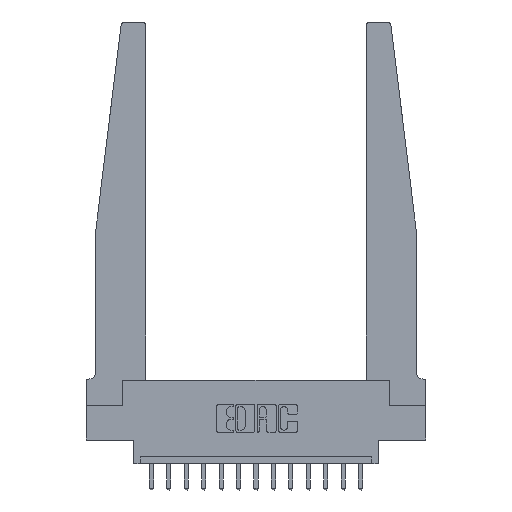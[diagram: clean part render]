
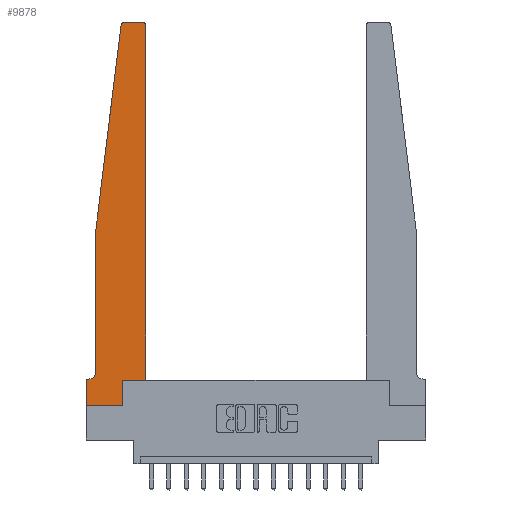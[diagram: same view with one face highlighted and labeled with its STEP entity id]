
A CAD part, top view. The second image highlights one B-rep face of the part: STEP entity #9878.
In plain terms, the highlighted planar face has unit normal (0, 0, 1).
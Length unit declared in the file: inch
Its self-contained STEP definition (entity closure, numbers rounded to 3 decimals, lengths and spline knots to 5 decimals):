
#317 = LINE ( 'NONE', #16357, #6888 ) ;
#931 = CARTESIAN_POINT ( 'NONE',  ( 0.015, 0.1875, 0.37 ) ) ;
#975 = EDGE_CURVE ( 'NONE', #17416, #9351, #16447, .T. ) ;
#1007 = DIRECTION ( 'NONE',  ( 1., 0., 0. ) ) ;
#1356 = VERTEX_POINT ( 'NONE', #2754 ) ;
#1375 = EDGE_CURVE ( 'NONE', #9351, #11897, #11931, .T. ) ;
#1663 = DIRECTION ( 'NONE',  ( -1., 0., 0. ) ) ;
#1745 = DIRECTION ( 'NONE',  ( 0., 0., -1. ) ) ;
#1753 = DIRECTION ( 'NONE',  ( 0., 0., 1. ) ) ;
#1827 = ORIENTED_EDGE ( 'NONE', *, *, #7842, .T. ) ;
#1927 = EDGE_CURVE ( 'NONE', #10220, #7853, #13602, .T. ) ;
#1990 = DIRECTION ( 'NONE',  ( 1., 0., 0. ) ) ;
#2330 = DIRECTION ( 'NONE',  ( 0., -1., 0. ) ) ;
#2385 = VERTEX_POINT ( 'NONE', #12582 ) ;
#2676 = EDGE_LOOP ( 'NONE', ( #6490, #8940, #11402, #15513, #10098, #4180, #11058, #1827, #3292, #8039, #5232, #17173 ) ) ;
#2754 = CARTESIAN_POINT ( 'NONE',  ( 0.425, 0.18, 0.37 ) ) ;
#2849 = VERTEX_POINT ( 'NONE', #7495 ) ;
#2889 = CARTESIAN_POINT ( 'NONE',  ( 0.2605, 0.18, 0.37 ) ) ;
#3292 = ORIENTED_EDGE ( 'NONE', *, *, #6015, .T. ) ;
#4180 = ORIENTED_EDGE ( 'NONE', *, *, #13503, .T. ) ;
#4207 = DIRECTION ( 'NONE',  ( 0., 1., 0. ) ) ;
#4223 = LINE ( 'NONE', #2889, #10040 ) ;
#4367 = VECTOR ( 'NONE', #1007, 39.37008 ) ;
#4486 = VERTEX_POINT ( 'NONE', #10503 ) ;
#4668 = FACE_OUTER_BOUND ( 'NONE', #2676, .T. ) ;
#5232 = ORIENTED_EDGE ( 'NONE', *, *, #15685, .T. ) ;
#5242 = DIRECTION ( 'NONE',  ( -1., 0., 0. ) ) ;
#5994 = AXIS2_PLACEMENT_3D ( 'NONE', #13742, #1745, #1663 ) ;
#6015 = EDGE_CURVE ( 'NONE', #2849, #12527, #4223, .T. ) ;
#6255 = CARTESIAN_POINT ( 'NONE',  ( 0.065, 1.25, 0.37 ) ) ;
#6296 = DIRECTION ( 'NONE',  ( 0., 0., 1. ) ) ;
#6426 = LINE ( 'NONE', #10212, #15548 ) ;
#6455 = DIRECTION ( 'NONE',  ( -0.122, -0.992, 0. ) ) ;
#6490 = ORIENTED_EDGE ( 'NONE', *, *, #13699, .T. ) ;
#6590 = EDGE_CURVE ( 'NONE', #4486, #8079, #13773, .T. ) ;
#6725 = CARTESIAN_POINT ( 'NONE',  ( 0.25, 2.75, 0.37 ) ) ;
#6888 = VECTOR ( 'NONE', #4207, 39.37008 ) ;
#7177 = CARTESIAN_POINT ( 'NONE',  ( 0., 0., 0.37 ) ) ;
#7495 = CARTESIAN_POINT ( 'NONE',  ( 0.2605, 0., 0.37 ) ) ;
#7842 = EDGE_CURVE ( 'NONE', #2385, #2849, #11161, .T. ) ;
#7853 = VERTEX_POINT ( 'NONE', #931 ) ;
#7958 = EDGE_CURVE ( 'NONE', #17322, #2385, #11512, .T. ) ;
#8039 = ORIENTED_EDGE ( 'NONE', *, *, #15219, .T. ) ;
#8075 = DIRECTION ( 'NONE',  ( -1., 0., 0. ) ) ;
#8079 = VERTEX_POINT ( 'NONE', #10423 ) ;
#8200 = AXIS2_PLACEMENT_3D ( 'NONE', #8365, #1753, #14012 ) ;
#8219 = DIRECTION ( 'NONE',  ( 1., 0., 0. ) ) ;
#8365 = CARTESIAN_POINT ( 'NONE',  ( 0., 0.1875, 0.37 ) ) ;
#8443 = VECTOR ( 'NONE', #1990, 39.37008 ) ;
#8846 = CARTESIAN_POINT ( 'NONE',  ( 0.425, 0.18, 0.37 ) ) ;
#8940 = ORIENTED_EDGE ( 'NONE', *, *, #975, .T. ) ;
#9100 = VECTOR ( 'NONE', #8075, 39.37008 ) ;
#9351 = VERTEX_POINT ( 'NONE', #9607 ) ;
#9607 = CARTESIAN_POINT ( 'NONE',  ( 0.24675, 2.72367, 0.37 ) ) ;
#9849 = PLANE ( 'NONE',  #8200 ) ;
#9878 = ADVANCED_FACE ( 'NONE', ( #4668 ), #9849, .T. ) ;
#9993 = EDGE_CURVE ( 'NONE', #11897, #10220, #6426, .T. ) ;
#10040 = VECTOR ( 'NONE', #16294, 39.37008 ) ;
#10098 = ORIENTED_EDGE ( 'NONE', *, *, #1927, .T. ) ;
#10212 = CARTESIAN_POINT ( 'NONE',  ( 0.065, 1.25, 0.37 ) ) ;
#10220 = VERTEX_POINT ( 'NONE', #10886 ) ;
#10389 = DIRECTION ( 'NONE',  ( 0., -1., 0. ) ) ;
#10423 = CARTESIAN_POINT ( 'NONE',  ( 0.395, 2.75, 0.37 ) ) ;
#10503 = CARTESIAN_POINT ( 'NONE',  ( 0.425, 2.72, 0.37 ) ) ;
#10886 = CARTESIAN_POINT ( 'NONE',  ( 0.065, 0.2375, 0.37 ) ) ;
#10997 = VECTOR ( 'NONE', #2330, 39.37008 ) ;
#11058 = ORIENTED_EDGE ( 'NONE', *, *, #7958, .T. ) ;
#11161 = LINE ( 'NONE', #7177, #8443 ) ;
#11402 = ORIENTED_EDGE ( 'NONE', *, *, #1375, .T. ) ;
#11512 = LINE ( 'NONE', #16885, #10997 ) ;
#11515 = CARTESIAN_POINT ( 'NONE',  ( 0.2605, 0.18, 0.37 ) ) ;
#11897 = VERTEX_POINT ( 'NONE', #6255 ) ;
#11931 = LINE ( 'NONE', #16062, #14258 ) ;
#12038 = CARTESIAN_POINT ( 'NONE',  ( 0., 0.1875, 0.37 ) ) ;
#12291 = DIRECTION ( 'NONE',  ( 0., 0., 1. ) ) ;
#12317 = LINE ( 'NONE', #16362, #9100 ) ;
#12465 = CARTESIAN_POINT ( 'NONE',  ( 0.27653, 2.75, 0.37 ) ) ;
#12527 = VERTEX_POINT ( 'NONE', #11515 ) ;
#12582 = CARTESIAN_POINT ( 'NONE',  ( 0., 0., 0.37 ) ) ;
#13362 = CARTESIAN_POINT ( 'NONE',  ( 0.27653, 2.72, 0.37 ) ) ;
#13503 = EDGE_CURVE ( 'NONE', #7853, #17322, #12317, .T. ) ;
#13602 = CIRCLE ( 'NONE', #5994, 0.05 ) ;
#13610 = LINE ( 'NONE', #6725, #15887 ) ;
#13699 = EDGE_CURVE ( 'NONE', #8079, #17416, #13610, .T. ) ;
#13742 = CARTESIAN_POINT ( 'NONE',  ( 0.015, 0.2375, 0.37 ) ) ;
#13773 = CIRCLE ( 'NONE', #14621, 0.03 ) ;
#13794 = CARTESIAN_POINT ( 'NONE',  ( 0.395, 2.72, 0.37 ) ) ;
#14012 = DIRECTION ( 'NONE',  ( 1., 0., 0. ) ) ;
#14236 = DIRECTION ( 'NONE',  ( 1., 0., 0. ) ) ;
#14258 = VECTOR ( 'NONE', #6455, 39.37008 ) ;
#14621 = AXIS2_PLACEMENT_3D ( 'NONE', #13794, #6296, #14236 ) ;
#15219 = EDGE_CURVE ( 'NONE', #12527, #1356, #16962, .T. ) ;
#15337 = AXIS2_PLACEMENT_3D ( 'NONE', #13362, #12291, #8219 ) ;
#15513 = ORIENTED_EDGE ( 'NONE', *, *, #9993, .T. ) ;
#15548 = VECTOR ( 'NONE', #10389, 39.37008 ) ;
#15685 = EDGE_CURVE ( 'NONE', #1356, #4486, #317, .T. ) ;
#15887 = VECTOR ( 'NONE', #5242, 39.37008 ) ;
#16062 = CARTESIAN_POINT ( 'NONE',  ( 0.065, 1.25, 0.37 ) ) ;
#16294 = DIRECTION ( 'NONE',  ( 0., 1., 0. ) ) ;
#16357 = CARTESIAN_POINT ( 'NONE',  ( 0.425, 0.18, 0.37 ) ) ;
#16362 = CARTESIAN_POINT ( 'NONE',  ( 0.065, 0.1875, 0.37 ) ) ;
#16447 = CIRCLE ( 'NONE', #15337, 0.03 ) ;
#16885 = CARTESIAN_POINT ( 'NONE',  ( 0., 0., 0.37 ) ) ;
#16962 = LINE ( 'NONE', #8846, #4367 ) ;
#17173 = ORIENTED_EDGE ( 'NONE', *, *, #6590, .T. ) ;
#17322 = VERTEX_POINT ( 'NONE', #12038 ) ;
#17416 = VERTEX_POINT ( 'NONE', #12465 ) ;
